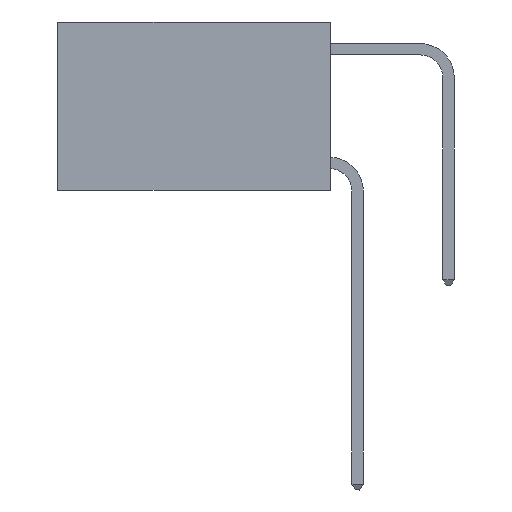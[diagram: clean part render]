
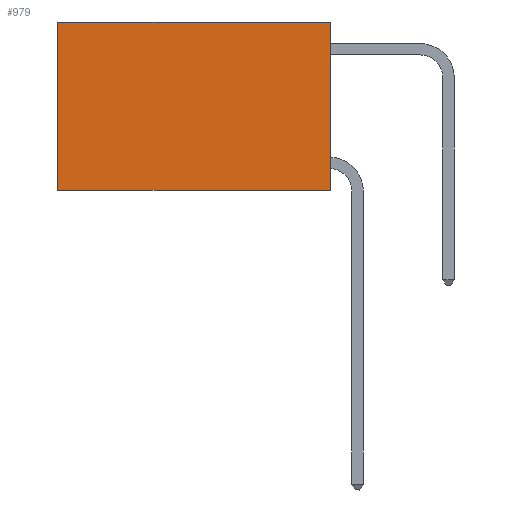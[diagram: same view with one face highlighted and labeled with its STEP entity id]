
A CAD part, left-side view. The second image highlights one B-rep face of the part: STEP entity #979.
In plain terms, the highlighted planar face has unit normal (-1, 0, 0).
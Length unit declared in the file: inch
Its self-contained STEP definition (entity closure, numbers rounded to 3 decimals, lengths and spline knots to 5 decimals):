
#118 = ORIENTED_EDGE ( 'NONE', *, *, #6317, .F. ) ;
#453 = EDGE_CURVE ( 'NONE', #13251, #3015, #9575, .T. ) ;
#979 = ADVANCED_FACE ( 'NONE', ( #2689 ), #12700, .F. ) ;
#1074 = VECTOR ( 'NONE', #12415, 39.37008 ) ;
#1116 = CARTESIAN_POINT ( 'NONE',  ( 0.2625, 0.6, 0. ) ) ;
#1714 = DIRECTION ( 'NONE',  ( 0., 1., 0. ) ) ;
#2533 = VECTOR ( 'NONE', #14134, 39.37008 ) ;
#2689 = FACE_OUTER_BOUND ( 'NONE', #9995, .T. ) ;
#3015 = VERTEX_POINT ( 'NONE', #9739 ) ;
#3373 = ORIENTED_EDGE ( 'NONE', *, *, #14101, .F. ) ;
#4082 = DIRECTION ( 'NONE',  ( 0., 0., -1. ) ) ;
#4273 = VECTOR ( 'NONE', #1714, 39.37008 ) ;
#4430 = CARTESIAN_POINT ( 'NONE',  ( 0.2625, 0., -0.37 ) ) ;
#5338 = CARTESIAN_POINT ( 'NONE',  ( 0.2625, 0., 0. ) ) ;
#6317 = EDGE_CURVE ( 'NONE', #12958, #3015, #8587, .T. ) ;
#6433 = ORIENTED_EDGE ( 'NONE', *, *, #11874, .T. ) ;
#6694 = VECTOR ( 'NONE', #11642, 39.37008 ) ;
#7174 = LINE ( 'NONE', #5338, #4273 ) ;
#8314 = LINE ( 'NONE', #11380, #1074 ) ;
#8587 = LINE ( 'NONE', #4430, #2533 ) ;
#9575 = LINE ( 'NONE', #13965, #6694 ) ;
#9652 = DIRECTION ( 'NONE',  ( 1., 0., 0. ) ) ;
#9739 = CARTESIAN_POINT ( 'NONE',  ( 0.2625, 0.6, -0.37 ) ) ;
#9866 = CARTESIAN_POINT ( 'NONE',  ( 0.2625, 0., -0.37 ) ) ;
#9995 = EDGE_LOOP ( 'NONE', ( #11834, #118, #3373, #6433 ) ) ;
#11380 = CARTESIAN_POINT ( 'NONE',  ( 0.2625, 0., 0. ) ) ;
#11642 = DIRECTION ( 'NONE',  ( 0., 0., -1. ) ) ;
#11834 = ORIENTED_EDGE ( 'NONE', *, *, #453, .T. ) ;
#11874 = EDGE_CURVE ( 'NONE', #13117, #13251, #7174, .T. ) ;
#12212 = CARTESIAN_POINT ( 'NONE',  ( 0.2625, 0., 0. ) ) ;
#12415 = DIRECTION ( 'NONE',  ( 0., 0., -1. ) ) ;
#12700 = PLANE ( 'NONE',  #13946 ) ;
#12958 = VERTEX_POINT ( 'NONE', #9866 ) ;
#13117 = VERTEX_POINT ( 'NONE', #13245 ) ;
#13245 = CARTESIAN_POINT ( 'NONE',  ( 0.2625, 0., 0. ) ) ;
#13251 = VERTEX_POINT ( 'NONE', #1116 ) ;
#13946 = AXIS2_PLACEMENT_3D ( 'NONE', #12212, #9652, #4082 ) ;
#13965 = CARTESIAN_POINT ( 'NONE',  ( 0.2625, 0.6, 0. ) ) ;
#14101 = EDGE_CURVE ( 'NONE', #13117, #12958, #8314, .T. ) ;
#14134 = DIRECTION ( 'NONE',  ( 0., 1., 0. ) ) ;
